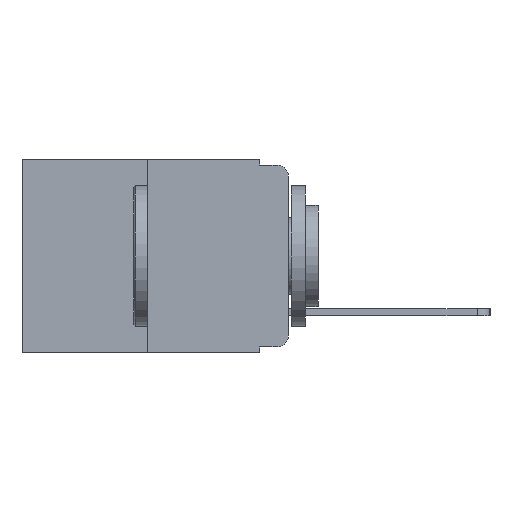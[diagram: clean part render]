
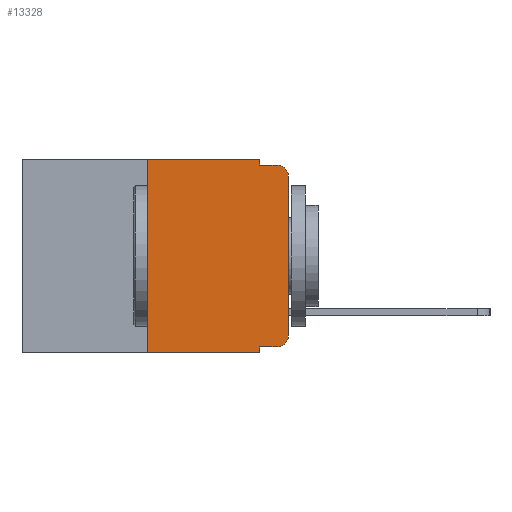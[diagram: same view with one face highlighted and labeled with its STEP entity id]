
A CAD part, left-side view. The second image highlights one B-rep face of the part: STEP entity #13328.
In plain terms, the highlighted planar face has unit normal (-1, 0, 0).
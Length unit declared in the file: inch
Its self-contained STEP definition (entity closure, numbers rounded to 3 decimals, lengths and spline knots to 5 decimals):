
#106 = ORIENTED_EDGE ( 'NONE', *, *, #8286, .T. ) ;
#513 = VERTEX_POINT ( 'NONE', #12921 ) ;
#579 = ORIENTED_EDGE ( 'NONE', *, *, #4835, .T. ) ;
#645 = AXIS2_PLACEMENT_3D ( 'NONE', #2178, #10788, #3489 ) ;
#777 = VERTEX_POINT ( 'NONE', #12738 ) ;
#1268 = ORIENTED_EDGE ( 'NONE', *, *, #12038, .T. ) ;
#1346 = EDGE_LOOP ( 'NONE', ( #1268, #2141, #14701, #5906, #12199, #12537, #106, #3762, #579, #5327 ) ) ;
#1356 = PLANE ( 'NONE',  #4044 ) ;
#1607 = EDGE_CURVE ( 'NONE', #513, #13586, #11788, .T. ) ;
#1713 = CARTESIAN_POINT ( 'NONE',  ( 0., 0.051, 0. ) ) ;
#2141 = ORIENTED_EDGE ( 'NONE', *, *, #11304, .T. ) ;
#2178 = CARTESIAN_POINT ( 'NONE',  ( 0., 0.02, -0.03 ) ) ;
#2242 = LINE ( 'NONE', #5085, #14471 ) ;
#2576 = VECTOR ( 'NONE', #6034, 39.37008 ) ;
#2727 = DIRECTION ( 'NONE',  ( 1., 0., 0. ) ) ;
#2886 = DIRECTION ( 'NONE',  ( 0., -1., 0. ) ) ;
#3017 = DIRECTION ( 'NONE',  ( -1., 0., 0. ) ) ;
#3470 = CARTESIAN_POINT ( 'NONE',  ( 0., 0., -0.03 ) ) ;
#3489 = DIRECTION ( 'NONE',  ( 0., 0., -1. ) ) ;
#3493 = VERTEX_POINT ( 'NONE', #7620 ) ;
#3762 = ORIENTED_EDGE ( 'NONE', *, *, #6524, .F. ) ;
#3764 = VECTOR ( 'NONE', #10994, 39.37008 ) ;
#3985 = VECTOR ( 'NONE', #15370, 39.37008 ) ;
#3996 = EDGE_CURVE ( 'NONE', #4123, #8309, #12126, .T. ) ;
#4044 = AXIS2_PLACEMENT_3D ( 'NONE', #11206, #2727, #11260 ) ;
#4123 = VERTEX_POINT ( 'NONE', #9575 ) ;
#4137 = AXIS2_PLACEMENT_3D ( 'NONE', #10399, #3017, #11512 ) ;
#4337 = VERTEX_POINT ( 'NONE', #5151 ) ;
#4835 = EDGE_CURVE ( 'NONE', #3493, #4123, #9486, .T. ) ;
#5085 = CARTESIAN_POINT ( 'NONE',  ( 0., 0.473, -0.343 ) ) ;
#5151 = CARTESIAN_POINT ( 'NONE',  ( 0., 0.051, -0.01 ) ) ;
#5327 = ORIENTED_EDGE ( 'NONE', *, *, #3996, .T. ) ;
#5413 = VECTOR ( 'NONE', #9635, 39.37008 ) ;
#5698 = CARTESIAN_POINT ( 'NONE',  ( 0., 0.25, -0.343 ) ) ;
#5906 = ORIENTED_EDGE ( 'NONE', *, *, #9034, .F. ) ;
#6034 = DIRECTION ( 'NONE',  ( 0., 0., -1. ) ) ;
#6524 = EDGE_CURVE ( 'NONE', #3493, #777, #8868, .T. ) ;
#7105 = LINE ( 'NONE', #8688, #3764 ) ;
#7150 = CARTESIAN_POINT ( 'NONE',  ( 0., 0.25, 0. ) ) ;
#7370 = VERTEX_POINT ( 'NONE', #3470 ) ;
#7371 = EDGE_CURVE ( 'NONE', #12707, #513, #8758, .T. ) ;
#7375 = CARTESIAN_POINT ( 'NONE',  ( 0., 0.473, 0. ) ) ;
#7540 = DIRECTION ( 'NONE',  ( 0., -1., 0. ) ) ;
#7620 = CARTESIAN_POINT ( 'NONE',  ( 0., 0.051, -0.333 ) ) ;
#8016 = DIRECTION ( 'NONE',  ( 0., 0., -1. ) ) ;
#8045 = FACE_OUTER_BOUND ( 'NONE', #1346, .T. ) ;
#8286 = EDGE_CURVE ( 'NONE', #12707, #777, #2242, .T. ) ;
#8309 = VERTEX_POINT ( 'NONE', #10289 ) ;
#8688 = CARTESIAN_POINT ( 'NONE',  ( 0., 0., 0. ) ) ;
#8758 = LINE ( 'NONE', #7150, #5413 ) ;
#8868 = LINE ( 'NONE', #13041, #2576 ) ;
#9034 = EDGE_CURVE ( 'NONE', #13586, #4337, #15594, .T. ) ;
#9250 = CIRCLE ( 'NONE', #645, 0.02 ) ;
#9486 = LINE ( 'NONE', #13383, #14916 ) ;
#9575 = CARTESIAN_POINT ( 'NONE',  ( 0., 0.02, -0.333 ) ) ;
#9635 = DIRECTION ( 'NONE',  ( 0., 0., 1. ) ) ;
#10241 = VERTEX_POINT ( 'NONE', #13023 ) ;
#10289 = CARTESIAN_POINT ( 'NONE',  ( 0., 0., -0.313 ) ) ;
#10399 = CARTESIAN_POINT ( 'NONE',  ( 0., 0.02, -0.313 ) ) ;
#10548 = EDGE_CURVE ( 'NONE', #4337, #10241, #13732, .T. ) ;
#10788 = DIRECTION ( 'NONE',  ( -1., 0., 0. ) ) ;
#10994 = DIRECTION ( 'NONE',  ( 0., 0., 1. ) ) ;
#11206 = CARTESIAN_POINT ( 'NONE',  ( 0., 0.473, 0. ) ) ;
#11260 = DIRECTION ( 'NONE',  ( 0., 0., -1. ) ) ;
#11304 = EDGE_CURVE ( 'NONE', #7370, #10241, #9250, .T. ) ;
#11449 = VECTOR ( 'NONE', #7540, 39.37008 ) ;
#11512 = DIRECTION ( 'NONE',  ( 0., 0., -1. ) ) ;
#11788 = LINE ( 'NONE', #7375, #11449 ) ;
#12038 = EDGE_CURVE ( 'NONE', #8309, #7370, #7105, .T. ) ;
#12126 = CIRCLE ( 'NONE', #4137, 0.02 ) ;
#12199 = ORIENTED_EDGE ( 'NONE', *, *, #1607, .F. ) ;
#12537 = ORIENTED_EDGE ( 'NONE', *, *, #7371, .F. ) ;
#12570 = CARTESIAN_POINT ( 'NONE',  ( 0., 0.051, 0. ) ) ;
#12707 = VERTEX_POINT ( 'NONE', #5698 ) ;
#12738 = CARTESIAN_POINT ( 'NONE',  ( 0., 0.051, -0.343 ) ) ;
#12762 = VECTOR ( 'NONE', #8016, 39.37008 ) ;
#12921 = CARTESIAN_POINT ( 'NONE',  ( 0., 0.25, 0. ) ) ;
#13023 = CARTESIAN_POINT ( 'NONE',  ( 0., 0.02, -0.01 ) ) ;
#13041 = CARTESIAN_POINT ( 'NONE',  ( 0., 0.051, 0. ) ) ;
#13291 = CARTESIAN_POINT ( 'NONE',  ( 0., 0.051, -0.01 ) ) ;
#13328 = ADVANCED_FACE ( 'NONE', ( #8045 ), #1356, .F. ) ;
#13383 = CARTESIAN_POINT ( 'NONE',  ( 0., 0.051, -0.333 ) ) ;
#13586 = VERTEX_POINT ( 'NONE', #1713 ) ;
#13732 = LINE ( 'NONE', #13291, #3985 ) ;
#14463 = DIRECTION ( 'NONE',  ( 0., -1., 0. ) ) ;
#14471 = VECTOR ( 'NONE', #2886, 39.37008 ) ;
#14701 = ORIENTED_EDGE ( 'NONE', *, *, #10548, .F. ) ;
#14916 = VECTOR ( 'NONE', #14463, 39.37008 ) ;
#15370 = DIRECTION ( 'NONE',  ( 0., -1., 0. ) ) ;
#15594 = LINE ( 'NONE', #12570, #12762 ) ;
